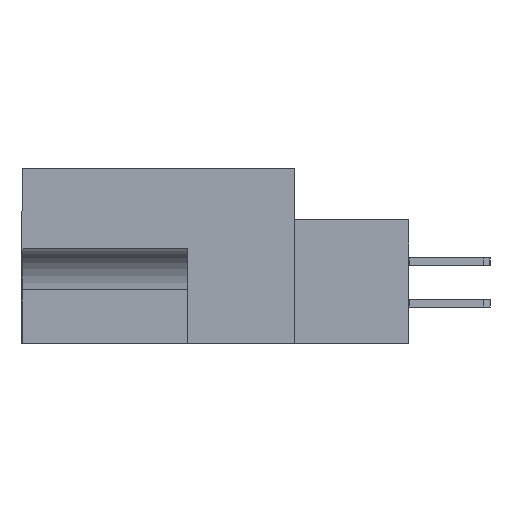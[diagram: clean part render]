
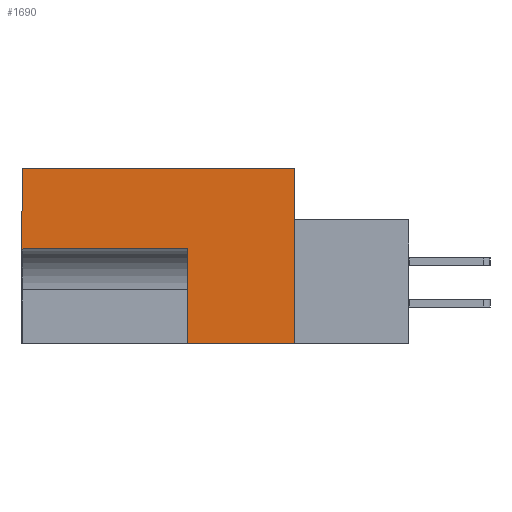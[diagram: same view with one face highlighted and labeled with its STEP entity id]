
A CAD part, left-side view. The second image highlights one B-rep face of the part: STEP entity #1690.
In plain terms, the highlighted planar face has unit normal (-1, 0, 0).
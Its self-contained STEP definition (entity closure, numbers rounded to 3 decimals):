
#1690 = ADVANCED_FACE ( 'NONE', ( #5393 ), #8053, .F. ) ;
#1802 = EDGE_CURVE ( 'NONE', #35732, #10515, #38018, .T. ) ;
#1840 = ORIENTED_EDGE ( 'NONE', *, *, #3705, .F. ) ;
#3705 = EDGE_CURVE ( 'NONE', #10515, #4795, #13025, .T. ) ;
#4287 = ORIENTED_EDGE ( 'NONE', *, *, #17569, .F. ) ;
#4755 = LINE ( 'NONE', #15170, #37402 ) ;
#4795 = VERTEX_POINT ( 'NONE', #11633 ) ;
#5393 = FACE_OUTER_BOUND ( 'NONE', #32513, .T. ) ;
#5741 = CARTESIAN_POINT ( 'NONE',  ( 0., 20.955, 0. ) ) ;
#6927 = ORIENTED_EDGE ( 'NONE', *, *, #40636, .F. ) ;
#8053 = PLANE ( 'NONE',  #33650 ) ;
#9144 = CARTESIAN_POINT ( 'NONE',  ( 0., 11.506, 0. ) ) ;
#9183 = CARTESIAN_POINT ( 'NONE',  ( 0., -8.814, -13.487 ) ) ;
#9801 = VERTEX_POINT ( 'NONE', #18311 ) ;
#10515 = VERTEX_POINT ( 'NONE', #38004 ) ;
#10810 = VECTOR ( 'NONE', #12359, 1000. ) ;
#11633 = CARTESIAN_POINT ( 'NONE',  ( 0., 0., -13.487 ) ) ;
#12359 = DIRECTION ( 'NONE',  ( 0., 0., 1. ) ) ;
#12674 = ORIENTED_EDGE ( 'NONE', *, *, #1802, .F. ) ;
#13025 = LINE ( 'NONE', #19590, #15979 ) ;
#13399 = CARTESIAN_POINT ( 'NONE',  ( 0., 8.255, -13.487 ) ) ;
#15170 = CARTESIAN_POINT ( 'NONE',  ( 0., 8.255, -6.172 ) ) ;
#15979 = VECTOR ( 'NONE', #22725, 1000. ) ;
#16706 = LINE ( 'NONE', #9183, #32076 ) ;
#17035 = ORIENTED_EDGE ( 'NONE', *, *, #22398, .F. ) ;
#17569 = EDGE_CURVE ( 'NONE', #37163, #35732, #27610, .T. ) ;
#17698 = DIRECTION ( 'NONE',  ( 1., 0., 0. ) ) ;
#18311 = CARTESIAN_POINT ( 'NONE',  ( 0., 8.255, -6.172 ) ) ;
#19590 = CARTESIAN_POINT ( 'NONE',  ( 0., 0., 0. ) ) ;
#19761 = DIRECTION ( 'NONE',  ( 0., 0., 1. ) ) ;
#19938 = CARTESIAN_POINT ( 'NONE',  ( 0., 8.255, -13.487 ) ) ;
#20499 = VECTOR ( 'NONE', #19761, 1000. ) ;
#21083 = DIRECTION ( 'NONE',  ( 0., 1., 0. ) ) ;
#21936 = ORIENTED_EDGE ( 'NONE', *, *, #39378, .F. ) ;
#22398 = EDGE_CURVE ( 'NONE', #4795, #31521, #16706, .T. ) ;
#22725 = DIRECTION ( 'NONE',  ( 0., 0., -1. ) ) ;
#26813 = DIRECTION ( 'NONE',  ( 0., 0., -1. ) ) ;
#27610 = LINE ( 'NONE', #37499, #10810 ) ;
#29919 = LINE ( 'NONE', #13399, #20499 ) ;
#31521 = VERTEX_POINT ( 'NONE', #19938 ) ;
#32076 = VECTOR ( 'NONE', #40934, 1000. ) ;
#32513 = EDGE_LOOP ( 'NONE', ( #17035, #1840, #12674, #4287, #21936, #6927 ) ) ;
#33187 = CARTESIAN_POINT ( 'NONE',  ( 0., 0., 0. ) ) ;
#33572 = VECTOR ( 'NONE', #37465, 1000. ) ;
#33650 = AXIS2_PLACEMENT_3D ( 'NONE', #33187, #17698, #26813 ) ;
#35732 = VERTEX_POINT ( 'NONE', #5741 ) ;
#37163 = VERTEX_POINT ( 'NONE', #37868 ) ;
#37402 = VECTOR ( 'NONE', #21083, 1000. ) ;
#37465 = DIRECTION ( 'NONE',  ( 0., -1., 0. ) ) ;
#37499 = CARTESIAN_POINT ( 'NONE',  ( 0., 20.955, -13.487 ) ) ;
#37868 = CARTESIAN_POINT ( 'NONE',  ( 0., 20.955, -6.172 ) ) ;
#38004 = CARTESIAN_POINT ( 'NONE',  ( 0., 0., 0. ) ) ;
#38018 = LINE ( 'NONE', #9144, #33572 ) ;
#39378 = EDGE_CURVE ( 'NONE', #9801, #37163, #4755, .T. ) ;
#40636 = EDGE_CURVE ( 'NONE', #31521, #9801, #29919, .T. ) ;
#40934 = DIRECTION ( 'NONE',  ( 0., 1., 0. ) ) ;
